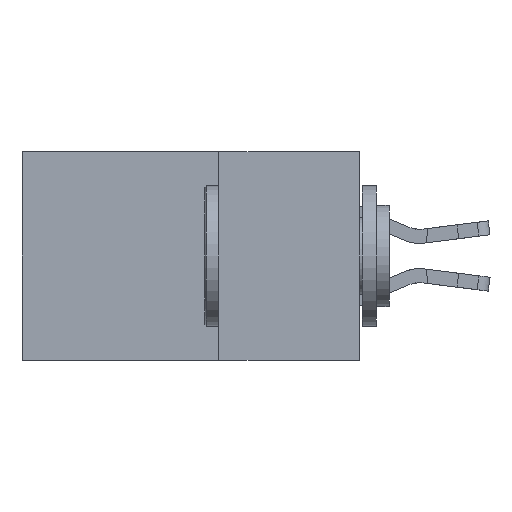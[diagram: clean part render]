
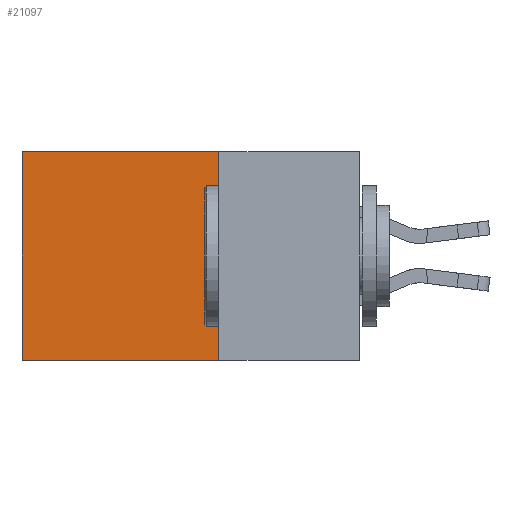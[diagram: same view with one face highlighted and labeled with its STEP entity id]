
A CAD part, left-side view. The second image highlights one B-rep face of the part: STEP entity #21097.
In plain terms, the highlighted planar face has unit normal (-1, 0, 0).
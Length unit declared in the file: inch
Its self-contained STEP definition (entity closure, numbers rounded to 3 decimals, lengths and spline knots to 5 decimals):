
#145 = CARTESIAN_POINT ( 'NONE',  ( 0.2875, 0.6, 0. ) ) ;
#2056 = ORIENTED_EDGE ( 'NONE', *, *, #10991, .T. ) ;
#2442 = EDGE_CURVE ( 'NONE', #9512, #17240, #7528, .T. ) ;
#4691 = CARTESIAN_POINT ( 'NONE',  ( 0.2875, 0.25, 0. ) ) ;
#5374 = LINE ( 'NONE', #11112, #21938 ) ;
#5604 = ORIENTED_EDGE ( 'NONE', *, *, #2442, .F. ) ;
#5614 = LINE ( 'NONE', #4691, #26272 ) ;
#5954 = PLANE ( 'NONE',  #22234 ) ;
#6455 = CARTESIAN_POINT ( 'NONE',  ( 0.2875, 0.25, 0. ) ) ;
#6879 = EDGE_LOOP ( 'NONE', ( #26486, #5604, #16441, #2056 ) ) ;
#6962 = EDGE_CURVE ( 'NONE', #26414, #17240, #14963, .T. ) ;
#7528 = LINE ( 'NONE', #17714, #18551 ) ;
#8102 = DIRECTION ( 'NONE',  ( 1., 0., 0. ) ) ;
#8178 = CARTESIAN_POINT ( 'NONE',  ( 0.2875, 0.25, -0.37 ) ) ;
#9224 = DIRECTION ( 'NONE',  ( 0., 0., -1. ) ) ;
#9512 = VERTEX_POINT ( 'NONE', #8178 ) ;
#10991 = EDGE_CURVE ( 'NONE', #23621, #26414, #5374, .T. ) ;
#11112 = CARTESIAN_POINT ( 'NONE',  ( 0.2875, 0.25, 0. ) ) ;
#14143 = CARTESIAN_POINT ( 'NONE',  ( 0.2875, 0.6, -0.37 ) ) ;
#14963 = LINE ( 'NONE', #23637, #24599 ) ;
#15451 = FACE_OUTER_BOUND ( 'NONE', #6879, .T. ) ;
#16441 = ORIENTED_EDGE ( 'NONE', *, *, #23742, .F. ) ;
#17197 = DIRECTION ( 'NONE',  ( 0., 0., -1. ) ) ;
#17240 = VERTEX_POINT ( 'NONE', #14143 ) ;
#17683 = DIRECTION ( 'NONE',  ( 0., 1., 0. ) ) ;
#17714 = CARTESIAN_POINT ( 'NONE',  ( 0.2875, 0.25, -0.37 ) ) ;
#18551 = VECTOR ( 'NONE', #17683, 39.37008 ) ;
#20495 = CARTESIAN_POINT ( 'NONE',  ( 0.2875, 0.25, 0. ) ) ;
#21097 = ADVANCED_FACE ( 'NONE', ( #15451 ), #5954, .F. ) ;
#21406 = DIRECTION ( 'NONE',  ( 0., 1., 0. ) ) ;
#21938 = VECTOR ( 'NONE', #21406, 39.37008 ) ;
#22234 = AXIS2_PLACEMENT_3D ( 'NONE', #20495, #8102, #22546 ) ;
#22546 = DIRECTION ( 'NONE',  ( 0., 0., -1. ) ) ;
#23621 = VERTEX_POINT ( 'NONE', #6455 ) ;
#23637 = CARTESIAN_POINT ( 'NONE',  ( 0.2875, 0.6, 0. ) ) ;
#23742 = EDGE_CURVE ( 'NONE', #23621, #9512, #5614, .T. ) ;
#24599 = VECTOR ( 'NONE', #9224, 39.37008 ) ;
#26272 = VECTOR ( 'NONE', #17197, 39.37008 ) ;
#26414 = VERTEX_POINT ( 'NONE', #145 ) ;
#26486 = ORIENTED_EDGE ( 'NONE', *, *, #6962, .T. ) ;
